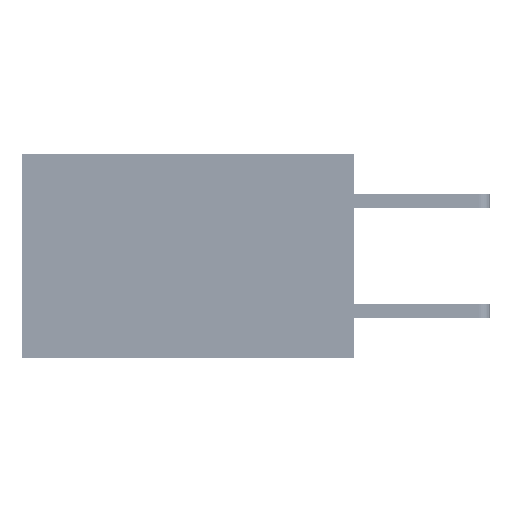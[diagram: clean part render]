
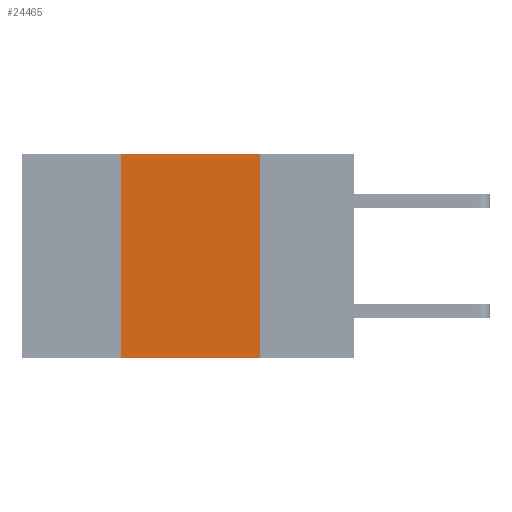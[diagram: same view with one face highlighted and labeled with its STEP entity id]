
A CAD part, left-side view. The second image highlights one B-rep face of the part: STEP entity #24465.
In plain terms, the highlighted planar face has unit normal (-1, 0, 0).
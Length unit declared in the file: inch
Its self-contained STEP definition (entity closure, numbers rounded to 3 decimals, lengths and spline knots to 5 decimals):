
#542 = CARTESIAN_POINT ( 'NONE',  ( 0., 0.6, -0.37 ) ) ;
#2598 = ORIENTED_EDGE ( 'NONE', *, *, #14939, .F. ) ;
#5014 = VERTEX_POINT ( 'NONE', #39841 ) ;
#5915 = LINE ( 'NONE', #38010, #32262 ) ;
#8523 = VECTOR ( 'NONE', #10500, 39.37008 ) ;
#9063 = VERTEX_POINT ( 'NONE', #24720 ) ;
#9297 = ORIENTED_EDGE ( 'NONE', *, *, #37831, .T. ) ;
#10500 = DIRECTION ( 'NONE',  ( 0., -1., 0. ) ) ;
#14357 = LINE ( 'NONE', #30640, #41710 ) ;
#14939 = EDGE_CURVE ( 'NONE', #9063, #24995, #14357, .T. ) ;
#16366 = EDGE_CURVE ( 'NONE', #24995, #23108, #27654, .T. ) ;
#18441 = CARTESIAN_POINT ( 'NONE',  ( 0., 0.6, 0. ) ) ;
#20390 = VECTOR ( 'NONE', #33918, 39.37008 ) ;
#23108 = VERTEX_POINT ( 'NONE', #27326 ) ;
#24465 = ADVANCED_FACE ( 'NONE', ( #36900 ), #25063, .F. ) ;
#24551 = EDGE_CURVE ( 'NONE', #23108, #5014, #5915, .T. ) ;
#24681 = CARTESIAN_POINT ( 'NONE',  ( 0., 0.6, 0. ) ) ;
#24720 = CARTESIAN_POINT ( 'NONE',  ( 0., 0.42, -0.37 ) ) ;
#24743 = ORIENTED_EDGE ( 'NONE', *, *, #16366, .F. ) ;
#24995 = VERTEX_POINT ( 'NONE', #36846 ) ;
#25063 = PLANE ( 'NONE',  #31021 ) ;
#27326 = CARTESIAN_POINT ( 'NONE',  ( 0., 0.17, 0. ) ) ;
#27630 = LINE ( 'NONE', #542, #8523 ) ;
#27654 = LINE ( 'NONE', #24681, #20390 ) ;
#28262 = DIRECTION ( 'NONE',  ( 1., 0., 0. ) ) ;
#28409 = DIRECTION ( 'NONE',  ( 0., 0., -1. ) ) ;
#28759 = EDGE_LOOP ( 'NONE', ( #29339, #24743, #2598, #9297 ) ) ;
#29339 = ORIENTED_EDGE ( 'NONE', *, *, #24551, .F. ) ;
#30640 = CARTESIAN_POINT ( 'NONE',  ( 0., 0.42, 0. ) ) ;
#31021 = AXIS2_PLACEMENT_3D ( 'NONE', #18441, #28262, #37869 ) ;
#32262 = VECTOR ( 'NONE', #28409, 39.37008 ) ;
#33918 = DIRECTION ( 'NONE',  ( 0., -1., 0. ) ) ;
#36846 = CARTESIAN_POINT ( 'NONE',  ( 0., 0.42, 0. ) ) ;
#36900 = FACE_OUTER_BOUND ( 'NONE', #28759, .T. ) ;
#37831 = EDGE_CURVE ( 'NONE', #9063, #5014, #27630, .T. ) ;
#37869 = DIRECTION ( 'NONE',  ( 0., 0., -1. ) ) ;
#38010 = CARTESIAN_POINT ( 'NONE',  ( 0., 0.17, 0. ) ) ;
#39841 = CARTESIAN_POINT ( 'NONE',  ( 0., 0.17, -0.37 ) ) ;
#40252 = DIRECTION ( 'NONE',  ( 0., 0., 1. ) ) ;
#41710 = VECTOR ( 'NONE', #40252, 39.37008 ) ;
